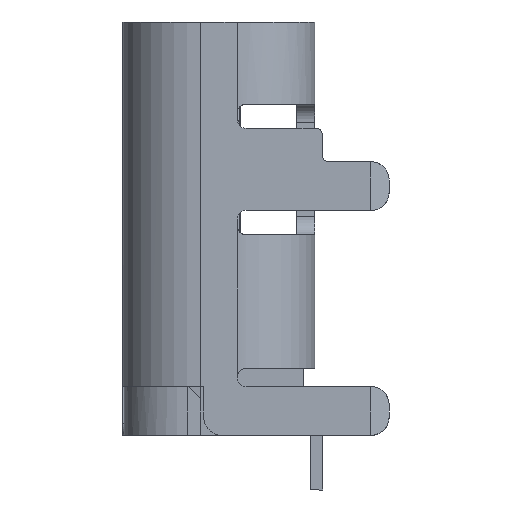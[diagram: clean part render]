
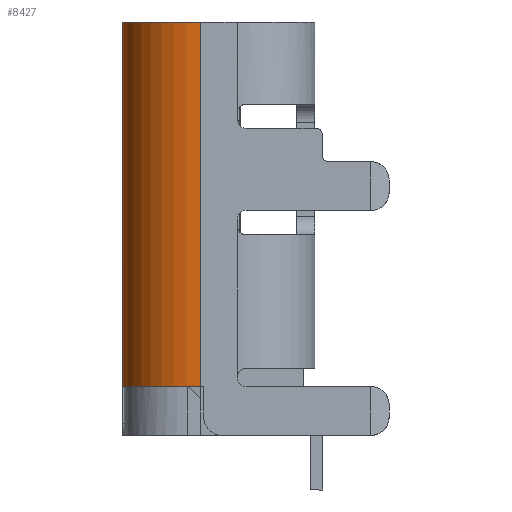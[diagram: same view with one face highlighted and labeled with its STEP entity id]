
A CAD part, left-side view. The second image highlights one B-rep face of the part: STEP entity #8427.
In plain terms, the highlighted cylindrical face has radius 1.28 mm (diameter 2.56 mm), a partial arc.
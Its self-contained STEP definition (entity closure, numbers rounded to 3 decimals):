
#126 = DIRECTION ( 'NONE',  ( 0., 1., 0. ) ) ;
#1127 = AXIS2_PLACEMENT_3D ( 'NONE', #11725, #126, #7896 ) ;
#1172 = CARTESIAN_POINT ( 'NONE',  ( -3.42, 5.1, 1.57 ) ) ;
#1421 = CARTESIAN_POINT ( 'NONE',  ( -3.19, 5.1, 1.591 ) ) ;
#1450 = VERTEX_POINT ( 'NONE', #6298 ) ;
#2760 = AXIS2_PLACEMENT_3D ( 'NONE', #5111, #6812, #4986 ) ;
#2834 = DIRECTION ( 'NONE',  ( 0., -1., 0. ) ) ;
#3085 = LINE ( 'NONE', #19154, #22832 ) ;
#3280 = CARTESIAN_POINT ( 'NONE',  ( -3.42, 5.1, 1.57 ) ) ;
#3393 = EDGE_LOOP ( 'NONE', ( #14982, #5936, #16469, #18232, #11799 ) ) ;
#3586 = CIRCLE ( 'NONE', #8199, 1.28 ) ;
#4650 = EDGE_CURVE ( 'NONE', #1450, #12704, #3085, .T. ) ;
#4906 = CIRCLE ( 'NONE', #1127, 1.28 ) ;
#4986 = DIRECTION ( 'NONE',  ( 0., 0., -1. ) ) ;
#5111 = CARTESIAN_POINT ( 'NONE',  ( -3.19, 5.357, 0.311 ) ) ;
#5936 = ORIENTED_EDGE ( 'NONE', *, *, #18074, .T. ) ;
#6298 = CARTESIAN_POINT ( 'NONE',  ( -3.19, 5.1, 1.591 ) ) ;
#6645 = EDGE_CURVE ( 'NONE', #14842, #17781, #23305, .T. ) ;
#6812 = DIRECTION ( 'NONE',  ( 0., -1., 0. ) ) ;
#7087 = CARTESIAN_POINT ( 'NONE',  ( -3.267, 5.1, 1.591 ) ) ;
#7896 = DIRECTION ( 'NONE',  ( 0., 0., -1. ) ) ;
#8199 = AXIS2_PLACEMENT_3D ( 'NONE', #17647, #15537, #9873 ) ;
#8427 = ADVANCED_FACE ( 'NONE', ( #11430 ), #19337, .T. ) ;
#9873 = DIRECTION ( 'NONE',  ( 0., 0., -1. ) ) ;
#9920 = CARTESIAN_POINT ( 'NONE',  ( -4.47, 5.1, 0.311 ) ) ;
#11366 = CARTESIAN_POINT ( 'NONE',  ( -4.47, -0.9, 0.311 ) ) ;
#11430 = FACE_OUTER_BOUND ( 'NONE', #3393, .T. ) ;
#11725 = CARTESIAN_POINT ( 'NONE',  ( -3.19, -0.9, 0.311 ) ) ;
#11799 = ORIENTED_EDGE ( 'NONE', *, *, #22779, .T. ) ;
#12704 = VERTEX_POINT ( 'NONE', #20183 ) ;
#14842 = VERTEX_POINT ( 'NONE', #9920 ) ;
#14982 = ORIENTED_EDGE ( 'NONE', *, *, #4650, .F. ) ;
#15232 = CARTESIAN_POINT ( 'NONE',  ( -3.344, 5.1, 1.584 ) ) ;
#15515 = DIRECTION ( 'NONE',  ( 0., -1., 0. ) ) ;
#15537 = DIRECTION ( 'NONE',  ( 0., -1., 0. ) ) ;
#16469 = ORIENTED_EDGE ( 'NONE', *, *, #19405, .T. ) ;
#17647 = CARTESIAN_POINT ( 'NONE',  ( -3.19, 5.1, 0.311 ) ) ;
#17781 = VERTEX_POINT ( 'NONE', #11366 ) ;
#18074 = EDGE_CURVE ( 'NONE', #1450, #18146, #21285, .T. ) ;
#18146 = VERTEX_POINT ( 'NONE', #3280 ) ;
#18232 = ORIENTED_EDGE ( 'NONE', *, *, #6645, .T. ) ;
#18703 = VECTOR ( 'NONE', #15515, 1000. ) ;
#19154 = CARTESIAN_POINT ( 'NONE',  ( -3.19, 2.5, 1.591 ) ) ;
#19337 = CYLINDRICAL_SURFACE ( 'NONE', #2760, 1.28 ) ;
#19405 = EDGE_CURVE ( 'NONE', #18146, #14842, #3586, .T. ) ;
#20183 = CARTESIAN_POINT ( 'NONE',  ( -3.19, -0.9, 1.591 ) ) ;
#21285 = B_SPLINE_CURVE_WITH_KNOTS ( 'NONE', 3,
 ( #1421, #7087, #15232, #1172 ),
 .UNSPECIFIED., .F., .F.,
 ( 4, 4 ),
 ( 0., 1. ),
 .UNSPECIFIED. ) ;
#22779 = EDGE_CURVE ( 'NONE', #17781, #12704, #4906, .T. ) ;
#22832 = VECTOR ( 'NONE', #2834, 1000. ) ;
#23305 = LINE ( 'NONE', #25412, #18703 ) ;
#25412 = CARTESIAN_POINT ( 'NONE',  ( -4.47, 5.357, 0.311 ) ) ;
